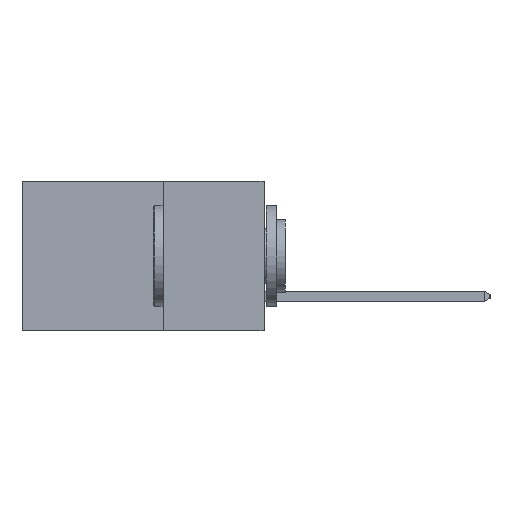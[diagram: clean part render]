
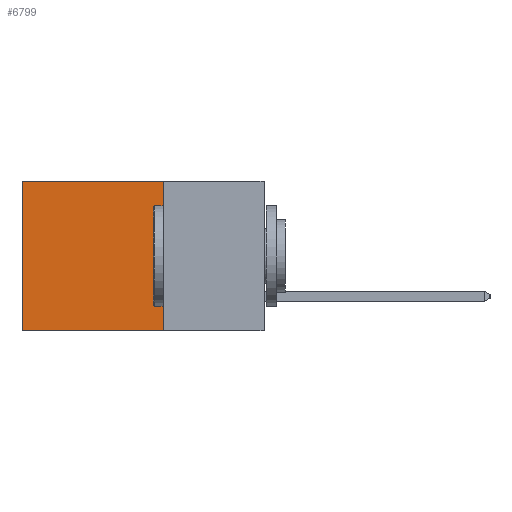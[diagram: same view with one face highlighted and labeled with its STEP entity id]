
A CAD part, left-side view. The second image highlights one B-rep face of the part: STEP entity #6799.
In plain terms, the highlighted planar face has unit normal (-1, 0, 0).
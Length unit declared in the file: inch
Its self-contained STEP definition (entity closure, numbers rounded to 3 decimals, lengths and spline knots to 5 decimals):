
#251 = VERTEX_POINT ( 'NONE', #17274 ) ;
#1167 = LINE ( 'NONE', #10836, #11664 ) ;
#2640 = EDGE_CURVE ( 'NONE', #10757, #9506, #2671, .T. ) ;
#2671 = LINE ( 'NONE', #4499, #12662 ) ;
#2883 = CARTESIAN_POINT ( 'NONE',  ( 0.2615, 0.6, 0. ) ) ;
#3039 = PLANE ( 'NONE',  #14061 ) ;
#4499 = CARTESIAN_POINT ( 'NONE',  ( 0.2615, 0.25, 0. ) ) ;
#4946 = ORIENTED_EDGE ( 'NONE', *, *, #2640, .T. ) ;
#5807 = DIRECTION ( 'NONE',  ( 0., 0., -1. ) ) ;
#5857 = CARTESIAN_POINT ( 'NONE',  ( 0.2615, 0.25, 0. ) ) ;
#6799 = ADVANCED_FACE ( 'NONE', ( #7625 ), #3039, .F. ) ;
#7043 = ORIENTED_EDGE ( 'NONE', *, *, #7566, .F. ) ;
#7566 = EDGE_CURVE ( 'NONE', #10757, #9924, #16448, .T. ) ;
#7625 = FACE_OUTER_BOUND ( 'NONE', #14288, .T. ) ;
#8768 = EDGE_CURVE ( 'NONE', #9506, #251, #14325, .T. ) ;
#9506 = VERTEX_POINT ( 'NONE', #2883 ) ;
#9563 = DIRECTION ( 'NONE',  ( 0., 1., 0. ) ) ;
#9924 = VERTEX_POINT ( 'NONE', #13503 ) ;
#10093 = DIRECTION ( 'NONE',  ( 0., 0., -1. ) ) ;
#10757 = VERTEX_POINT ( 'NONE', #5857 ) ;
#10836 = CARTESIAN_POINT ( 'NONE',  ( 0.2615, 0.25, -0.37 ) ) ;
#11266 = EDGE_CURVE ( 'NONE', #9924, #251, #1167, .T. ) ;
#11422 = CARTESIAN_POINT ( 'NONE',  ( 0.2615, 0.25, -0.37 ) ) ;
#11480 = DIRECTION ( 'NONE',  ( 0., 0., -1. ) ) ;
#11633 = ORIENTED_EDGE ( 'NONE', *, *, #8768, .T. ) ;
#11664 = VECTOR ( 'NONE', #9563, 39.37008 ) ;
#12440 = VECTOR ( 'NONE', #11480, 39.37008 ) ;
#12526 = CARTESIAN_POINT ( 'NONE',  ( 0.2615, 0.25, -0.37 ) ) ;
#12662 = VECTOR ( 'NONE', #17043, 39.37008 ) ;
#13503 = CARTESIAN_POINT ( 'NONE',  ( 0.2615, 0.25, -0.37 ) ) ;
#13717 = ORIENTED_EDGE ( 'NONE', *, *, #11266, .F. ) ;
#13887 = DIRECTION ( 'NONE',  ( 1., 0., 0. ) ) ;
#13903 = VECTOR ( 'NONE', #10093, 39.37008 ) ;
#14061 = AXIS2_PLACEMENT_3D ( 'NONE', #12526, #13887, #5807 ) ;
#14288 = EDGE_LOOP ( 'NONE', ( #11633, #13717, #7043, #4946 ) ) ;
#14325 = LINE ( 'NONE', #15488, #13903 ) ;
#15488 = CARTESIAN_POINT ( 'NONE',  ( 0.2615, 0.6, -0.37 ) ) ;
#16448 = LINE ( 'NONE', #11422, #12440 ) ;
#17043 = DIRECTION ( 'NONE',  ( 0., 1., 0. ) ) ;
#17274 = CARTESIAN_POINT ( 'NONE',  ( 0.2615, 0.6, -0.37 ) ) ;
